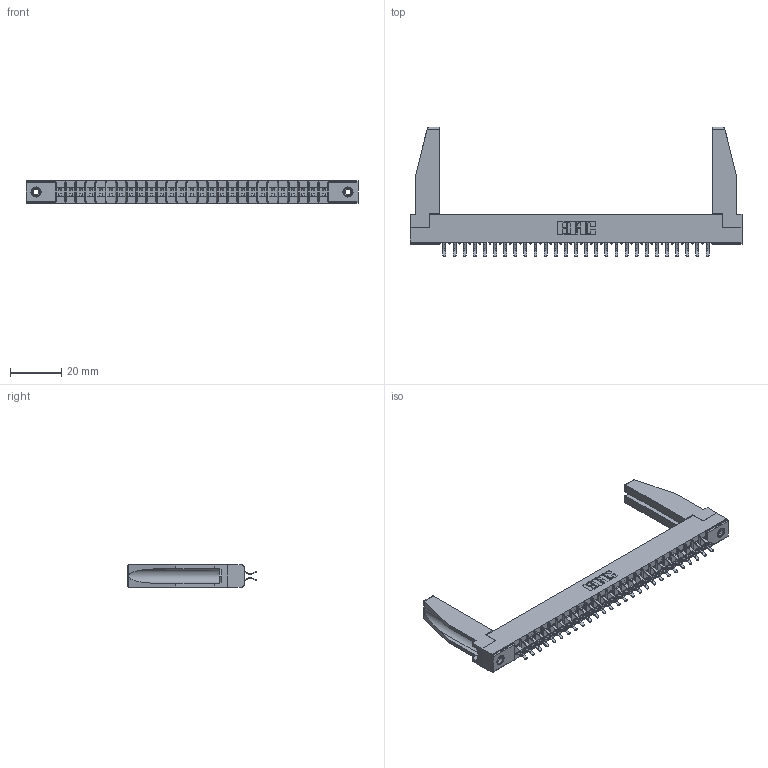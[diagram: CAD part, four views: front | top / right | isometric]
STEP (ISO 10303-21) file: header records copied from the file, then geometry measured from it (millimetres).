
FILE_DESCRIPTION (( 'STEP AP203' ), '1' );
FILE_NAME ('355-054-556-578.STEP', '2019-09-11T17:25:11', ( '' ), ( '' ), 'SwSTEP 2.0', 'SolidWorks 2016', '' );
FILE_SCHEMA (( 'CONFIG_CONTROL_DESIGN' ));
Length unit declared in the file: inch
Products named in the file (5): 305-290-001_556; 307-220-078; 305 Part_.156 Dia; 355-054-556-578; 345-250-001_345-250-001-102
Assembly tree (59 placements, depth 2):
  355-054-556-578
    305 Part_.156 Dia
    305-290-001_556  x54
    345-250-001_345-250-001-102  x2
    307-220-078  x2
Bounding box: 130 x 50.67 x 8.71 mm (x, y, z)
Volume: 11755.5 mm3; surface area: 19630.4 mm2
Topology: 59 solids, 59 shells, 3270 faces, 9367 edges, 6090 vertices
Faces by surface type: plane 1826, cylinder 1320, sphere 108, cone 12, torus 4
Entity records: 33721 total; most frequent: CARTESIAN_POINT 5589, ORIENTED_EDGE 5504, DIRECTION 5380, EDGE_CURVE 2752, LINE 2202, VECTOR 2202, VERTEX_POINT 1756, AXIS2_PLACEMENT_3D 1589
